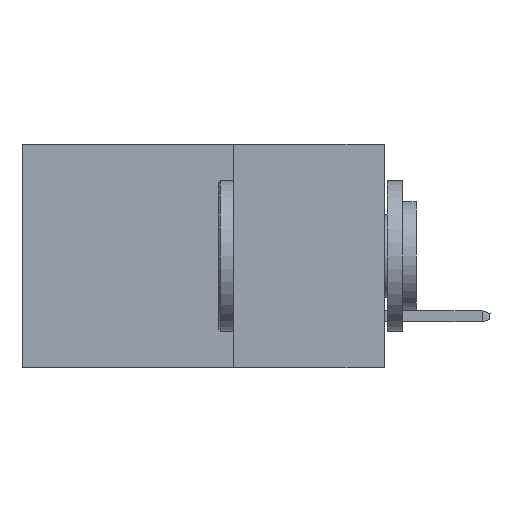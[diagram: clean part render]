
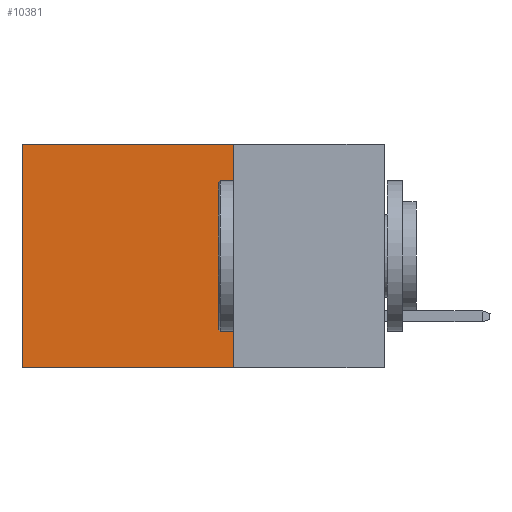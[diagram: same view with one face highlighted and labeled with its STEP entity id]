
A CAD part, left-side view. The second image highlights one B-rep face of the part: STEP entity #10381.
In plain terms, the highlighted planar face has unit normal (-1, 0, 0).
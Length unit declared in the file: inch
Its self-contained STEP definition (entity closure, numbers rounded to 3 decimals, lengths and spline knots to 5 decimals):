
#383 = EDGE_CURVE ( 'NONE', #3646, #10481, #12018, .T. ) ;
#472 = CARTESIAN_POINT ( 'NONE',  ( 0.298, 0.25, -0.37 ) ) ;
#806 = VECTOR ( 'NONE', #2026, 39.37008 ) ;
#1129 = DIRECTION ( 'NONE',  ( 0., 0., -1. ) ) ;
#1660 = ORIENTED_EDGE ( 'NONE', *, *, #2753, .F. ) ;
#2026 = DIRECTION ( 'NONE',  ( 0., 0., -1. ) ) ;
#2629 = AXIS2_PLACEMENT_3D ( 'NONE', #16486, #4954, #1129 ) ;
#2753 = EDGE_CURVE ( 'NONE', #6827, #13809, #7911, .T. ) ;
#3646 = VERTEX_POINT ( 'NONE', #10008 ) ;
#4350 = EDGE_CURVE ( 'NONE', #13809, #10481, #14327, .T. ) ;
#4550 = VECTOR ( 'NONE', #14219, 39.37008 ) ;
#4951 = EDGE_LOOP ( 'NONE', ( #14826, #10601, #1660, #5120 ) ) ;
#4954 = DIRECTION ( 'NONE',  ( 1., 0., 0. ) ) ;
#5015 = PLANE ( 'NONE',  #2629 ) ;
#5120 = ORIENTED_EDGE ( 'NONE', *, *, #10960, .T. ) ;
#5619 = LINE ( 'NONE', #11854, #15467 ) ;
#6640 = DIRECTION ( 'NONE',  ( 0., 1., 0. ) ) ;
#6827 = VERTEX_POINT ( 'NONE', #9753 ) ;
#7663 = CARTESIAN_POINT ( 'NONE',  ( 0.298, 0.25, 0. ) ) ;
#7911 = LINE ( 'NONE', #7663, #4550 ) ;
#9753 = CARTESIAN_POINT ( 'NONE',  ( 0.298, 0.25, 0. ) ) ;
#10008 = CARTESIAN_POINT ( 'NONE',  ( 0.298, 0.6, 0. ) ) ;
#10381 = ADVANCED_FACE ( 'NONE', ( #12694 ), #5015, .F. ) ;
#10481 = VERTEX_POINT ( 'NONE', #11282 ) ;
#10601 = ORIENTED_EDGE ( 'NONE', *, *, #4350, .F. ) ;
#10960 = EDGE_CURVE ( 'NONE', #6827, #3646, #5619, .T. ) ;
#11282 = CARTESIAN_POINT ( 'NONE',  ( 0.298, 0.6, -0.37 ) ) ;
#11854 = CARTESIAN_POINT ( 'NONE',  ( 0.298, 0.25, 0. ) ) ;
#12018 = LINE ( 'NONE', #16358, #806 ) ;
#12694 = FACE_OUTER_BOUND ( 'NONE', #4951, .T. ) ;
#13425 = DIRECTION ( 'NONE',  ( 0., 1., 0. ) ) ;
#13687 = CARTESIAN_POINT ( 'NONE',  ( 0.298, 0.25, -0.37 ) ) ;
#13809 = VERTEX_POINT ( 'NONE', #13687 ) ;
#13943 = VECTOR ( 'NONE', #13425, 39.37008 ) ;
#14219 = DIRECTION ( 'NONE',  ( 0., 0., -1. ) ) ;
#14327 = LINE ( 'NONE', #472, #13943 ) ;
#14826 = ORIENTED_EDGE ( 'NONE', *, *, #383, .T. ) ;
#15467 = VECTOR ( 'NONE', #6640, 39.37008 ) ;
#16358 = CARTESIAN_POINT ( 'NONE',  ( 0.298, 0.6, 0. ) ) ;
#16486 = CARTESIAN_POINT ( 'NONE',  ( 0.298, 0.25, 0. ) ) ;
